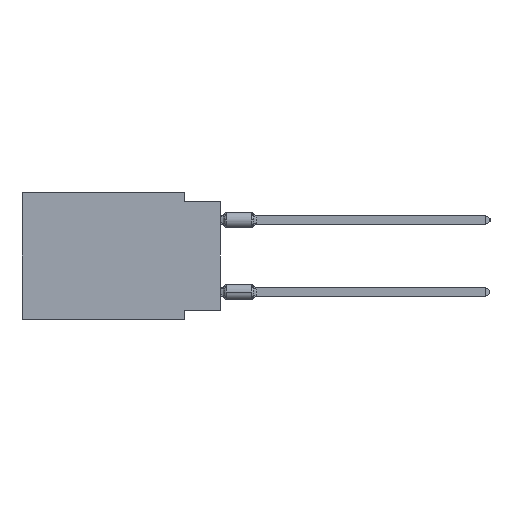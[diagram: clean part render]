
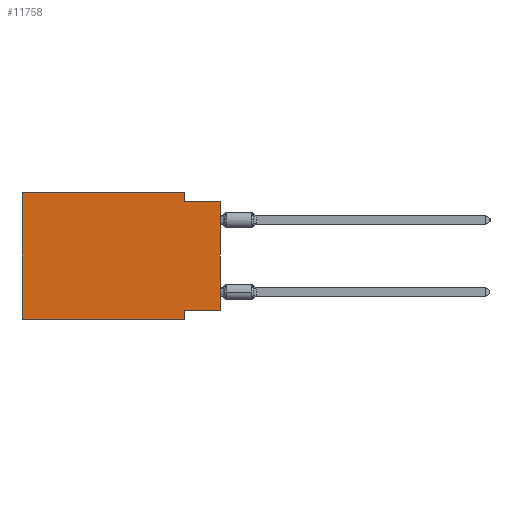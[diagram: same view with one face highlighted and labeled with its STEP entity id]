
A CAD part, left-side view. The second image highlights one B-rep face of the part: STEP entity #11758.
In plain terms, the highlighted planar face has unit normal (-1, 0, 0).
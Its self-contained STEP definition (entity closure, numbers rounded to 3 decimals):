
#1088 = CARTESIAN_POINT ( 'NONE',  ( 0., 2.54, 0. ) ) ;
#2158 = EDGE_CURVE ( 'NONE', #5753, #21158, #21279, .T. ) ;
#2566 = DIRECTION ( 'NONE',  ( 0., 0., 1. ) ) ;
#2578 = FACE_OUTER_BOUND ( 'NONE', #49480, .T. ) ;
#2593 = DIRECTION ( 'NONE',  ( 0., -1., 0. ) ) ;
#2937 = CARTESIAN_POINT ( 'NONE',  ( 0., 2.54, -8.255 ) ) ;
#3767 = VECTOR ( 'NONE', #15125, 1000. ) ;
#4441 = CARTESIAN_POINT ( 'NONE',  ( 0., 0., -0.635 ) ) ;
#5423 = ORIENTED_EDGE ( 'NONE', *, *, #17872, .T. ) ;
#5753 = VERTEX_POINT ( 'NONE', #41292 ) ;
#6970 = DIRECTION ( 'NONE',  ( 1., 0., 0. ) ) ;
#8083 = AXIS2_PLACEMENT_3D ( 'NONE', #25367, #6970, #51716 ) ;
#8602 = DIRECTION ( 'NONE',  ( 0., 0., 1. ) ) ;
#9922 = CARTESIAN_POINT ( 'NONE',  ( 0., 2.54, -8.89 ) ) ;
#11098 = CARTESIAN_POINT ( 'NONE',  ( 0., 0., -8.255 ) ) ;
#11758 = ADVANCED_FACE ( 'NONE', ( #2578 ), #56690, .F. ) ;
#12156 = CARTESIAN_POINT ( 'NONE',  ( 0., 2.54, -8.89 ) ) ;
#12410 = CARTESIAN_POINT ( 'NONE',  ( 0., 13.97, 0. ) ) ;
#14722 = ORIENTED_EDGE ( 'NONE', *, *, #2158, .F. ) ;
#15125 = DIRECTION ( 'NONE',  ( 0., -1., 0. ) ) ;
#15340 = VECTOR ( 'NONE', #45226, 1000. ) ;
#16381 = LINE ( 'NONE', #47942, #16573 ) ;
#16573 = VECTOR ( 'NONE', #20458, 1000. ) ;
#16795 = LINE ( 'NONE', #12410, #40498 ) ;
#17235 = LINE ( 'NONE', #35053, #41655 ) ;
#17872 = EDGE_CURVE ( 'NONE', #56921, #41319, #42633, .T. ) ;
#18123 = LINE ( 'NONE', #9922, #39205 ) ;
#18595 = EDGE_CURVE ( 'NONE', #46731, #5753, #16795, .T. ) ;
#20012 = VECTOR ( 'NONE', #2566, 1000. ) ;
#20458 = DIRECTION ( 'NONE',  ( 0., -1., 0. ) ) ;
#20909 = ORIENTED_EDGE ( 'NONE', *, *, #50411, .F. ) ;
#21158 = VERTEX_POINT ( 'NONE', #26635 ) ;
#21279 = LINE ( 'NONE', #30075, #43730 ) ;
#25367 = CARTESIAN_POINT ( 'NONE',  ( 0., 13.97, 0. ) ) ;
#26635 = CARTESIAN_POINT ( 'NONE',  ( 0., 2.54, 0. ) ) ;
#27102 = ORIENTED_EDGE ( 'NONE', *, *, #54166, .F. ) ;
#27182 = VERTEX_POINT ( 'NONE', #2937 ) ;
#27396 = LINE ( 'NONE', #1088, #15340 ) ;
#27405 = EDGE_CURVE ( 'NONE', #56921, #27182, #17235, .T. ) ;
#27723 = VERTEX_POINT ( 'NONE', #39088 ) ;
#27988 = LINE ( 'NONE', #46403, #3767 ) ;
#30075 = CARTESIAN_POINT ( 'NONE',  ( 0., 13.97, 0. ) ) ;
#30569 = EDGE_CURVE ( 'NONE', #46731, #51015, #16381, .T. ) ;
#30615 = CARTESIAN_POINT ( 'NONE',  ( 0., 0., 0. ) ) ;
#32953 = CARTESIAN_POINT ( 'NONE',  ( 0., 13.97, -8.89 ) ) ;
#35053 = CARTESIAN_POINT ( 'NONE',  ( 0., 0., -8.255 ) ) ;
#39088 = CARTESIAN_POINT ( 'NONE',  ( 0., 2.54, -0.635 ) ) ;
#39205 = VECTOR ( 'NONE', #53807, 1000. ) ;
#39883 = ORIENTED_EDGE ( 'NONE', *, *, #27405, .F. ) ;
#40498 = VECTOR ( 'NONE', #8602, 1000. ) ;
#41292 = CARTESIAN_POINT ( 'NONE',  ( 0., 13.97, 0. ) ) ;
#41319 = VERTEX_POINT ( 'NONE', #4441 ) ;
#41655 = VECTOR ( 'NONE', #52912, 1000. ) ;
#42633 = LINE ( 'NONE', #30615, #20012 ) ;
#43730 = VECTOR ( 'NONE', #2593, 1000. ) ;
#44282 = ORIENTED_EDGE ( 'NONE', *, *, #30569, .T. ) ;
#45226 = DIRECTION ( 'NONE',  ( 0., 0., -1. ) ) ;
#46403 = CARTESIAN_POINT ( 'NONE',  ( 0., 0., -0.635 ) ) ;
#46731 = VERTEX_POINT ( 'NONE', #32953 ) ;
#47764 = ORIENTED_EDGE ( 'NONE', *, *, #57393, .F. ) ;
#47942 = CARTESIAN_POINT ( 'NONE',  ( 0., 13.97, -8.89 ) ) ;
#49480 = EDGE_LOOP ( 'NONE', ( #5423, #47764, #27102, #14722, #56259, #44282, #20909, #39883 ) ) ;
#50411 = EDGE_CURVE ( 'NONE', #27182, #51015, #18123, .T. ) ;
#51015 = VERTEX_POINT ( 'NONE', #12156 ) ;
#51716 = DIRECTION ( 'NONE',  ( 0., 0., -1. ) ) ;
#52912 = DIRECTION ( 'NONE',  ( 0., 1., 0. ) ) ;
#53807 = DIRECTION ( 'NONE',  ( 0., 0., -1. ) ) ;
#54166 = EDGE_CURVE ( 'NONE', #21158, #27723, #27396, .T. ) ;
#56259 = ORIENTED_EDGE ( 'NONE', *, *, #18595, .F. ) ;
#56690 = PLANE ( 'NONE',  #8083 ) ;
#56921 = VERTEX_POINT ( 'NONE', #11098 ) ;
#57393 = EDGE_CURVE ( 'NONE', #27723, #41319, #27988, .T. ) ;
